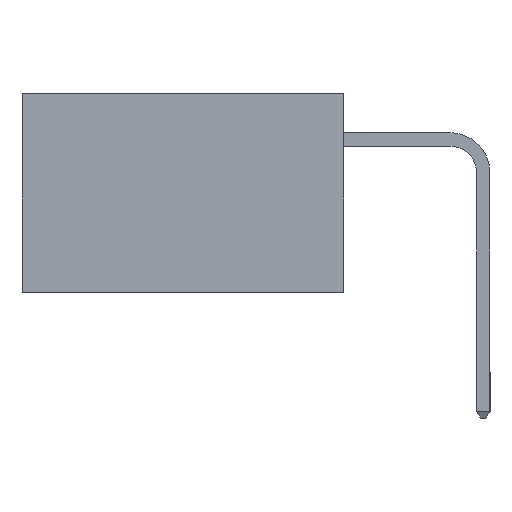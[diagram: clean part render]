
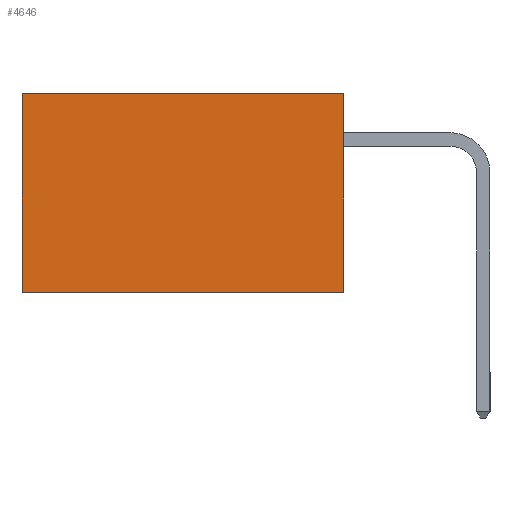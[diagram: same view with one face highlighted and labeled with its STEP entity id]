
A CAD part, left-side view. The second image highlights one B-rep face of the part: STEP entity #4646.
In plain terms, the highlighted planar face has unit normal (-1, 0, 0).
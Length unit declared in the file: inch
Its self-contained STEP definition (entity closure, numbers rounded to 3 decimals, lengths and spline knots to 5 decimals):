
#93 = LINE ( 'NONE', #3391, #10462 ) ;
#110 = CARTESIAN_POINT ( 'NONE',  ( 0.2615, 0., 0. ) ) ;
#379 = CARTESIAN_POINT ( 'NONE',  ( 0.2615, 0.6, -0.37 ) ) ;
#456 = ORIENTED_EDGE ( 'NONE', *, *, #1642, .F. ) ;
#737 = LINE ( 'NONE', #3206, #9350 ) ;
#739 = ORIENTED_EDGE ( 'NONE', *, *, #3952, .F. ) ;
#1150 = EDGE_CURVE ( 'NONE', #6327, #5419, #737, .T. ) ;
#1198 = ORIENTED_EDGE ( 'NONE', *, *, #2704, .T. ) ;
#1460 = DIRECTION ( 'NONE',  ( 0., 0., -1. ) ) ;
#1642 = EDGE_CURVE ( 'NONE', #8862, #3189, #10261, .T. ) ;
#1817 = DIRECTION ( 'NONE',  ( 0., 1., 0. ) ) ;
#2133 = AXIS2_PLACEMENT_3D ( 'NONE', #8828, #2559, #4792 ) ;
#2559 = DIRECTION ( 'NONE',  ( 1., 0., 0. ) ) ;
#2704 = EDGE_CURVE ( 'NONE', #8862, #6327, #5184, .T. ) ;
#2908 = EDGE_LOOP ( 'NONE', ( #5532, #739, #456, #1198 ) ) ;
#3189 = VERTEX_POINT ( 'NONE', #3526 ) ;
#3206 = CARTESIAN_POINT ( 'NONE',  ( 0.2615, 0.6, -0.37 ) ) ;
#3391 = CARTESIAN_POINT ( 'NONE',  ( 0.2615, 0., -0.37 ) ) ;
#3526 = CARTESIAN_POINT ( 'NONE',  ( 0.2615, 0., -0.37 ) ) ;
#3952 = EDGE_CURVE ( 'NONE', #3189, #5419, #93, .T. ) ;
#4646 = ADVANCED_FACE ( 'NONE', ( #9635 ), #10537, .F. ) ;
#4792 = DIRECTION ( 'NONE',  ( 0., 0., -1. ) ) ;
#5184 = LINE ( 'NONE', #9116, #7361 ) ;
#5419 = VERTEX_POINT ( 'NONE', #379 ) ;
#5532 = ORIENTED_EDGE ( 'NONE', *, *, #1150, .T. ) ;
#5556 = DIRECTION ( 'NONE',  ( 0., 0., -1. ) ) ;
#6094 = CARTESIAN_POINT ( 'NONE',  ( 0.2615, 0.6, 0. ) ) ;
#6327 = VERTEX_POINT ( 'NONE', #6094 ) ;
#6626 = DIRECTION ( 'NONE',  ( 0., 1., 0. ) ) ;
#7361 = VECTOR ( 'NONE', #1817, 39.37008 ) ;
#8532 = VECTOR ( 'NONE', #1460, 39.37008 ) ;
#8727 = CARTESIAN_POINT ( 'NONE',  ( 0.2615, 0., -0.37 ) ) ;
#8828 = CARTESIAN_POINT ( 'NONE',  ( 0.2615, 0., -0.37 ) ) ;
#8862 = VERTEX_POINT ( 'NONE', #110 ) ;
#9116 = CARTESIAN_POINT ( 'NONE',  ( 0.2615, 0., 0. ) ) ;
#9350 = VECTOR ( 'NONE', #5556, 39.37008 ) ;
#9635 = FACE_OUTER_BOUND ( 'NONE', #2908, .T. ) ;
#10261 = LINE ( 'NONE', #8727, #8532 ) ;
#10462 = VECTOR ( 'NONE', #6626, 39.37008 ) ;
#10537 = PLANE ( 'NONE',  #2133 ) ;
